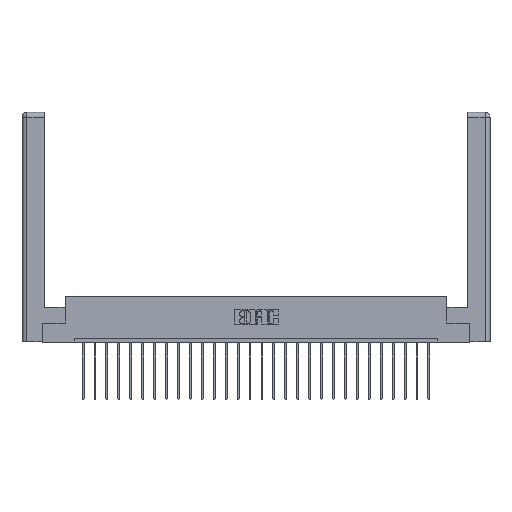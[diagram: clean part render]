
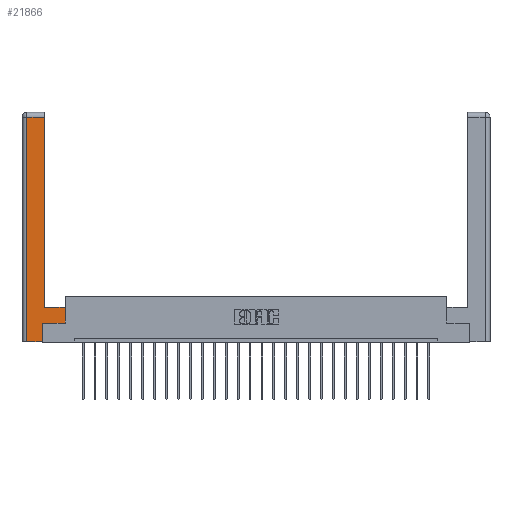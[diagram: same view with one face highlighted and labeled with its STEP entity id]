
A CAD part, top view. The second image highlights one B-rep face of the part: STEP entity #21866.
In plain terms, the highlighted planar face has unit normal (0, 0, 1).
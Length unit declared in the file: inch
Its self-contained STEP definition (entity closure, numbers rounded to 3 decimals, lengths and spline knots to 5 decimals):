
#73 = EDGE_CURVE ( 'NONE', #23900, #25314, #4534, .T. ) ;
#271 = CARTESIAN_POINT ( 'NONE',  ( 0.295, 0.45, 0. ) ) ;
#845 = VECTOR ( 'NONE', #26186, 39.37008 ) ;
#1394 = EDGE_LOOP ( 'NONE', ( #19940, #19901, #8813, #25549, #12330, #16072, #11205, #23331 ) ) ;
#1523 = CARTESIAN_POINT ( 'NONE',  ( 0.565, 0.245, 0. ) ) ;
#1607 = AXIS2_PLACEMENT_3D ( 'NONE', #14791, #22814, #22998 ) ;
#3535 = CARTESIAN_POINT ( 'NONE',  ( 0.265, 0.245, 0. ) ) ;
#4013 = DIRECTION ( 'NONE',  ( -1., 0., 0. ) ) ;
#4534 = LINE ( 'NONE', #16246, #7686 ) ;
#4555 = VECTOR ( 'NONE', #17976, 39.37008 ) ;
#5051 = EDGE_CURVE ( 'NONE', #6829, #8769, #17797, .T. ) ;
#5278 = EDGE_CURVE ( 'NONE', #17995, #23900, #6553, .T. ) ;
#5925 = DIRECTION ( 'NONE',  ( 0., 1., 0. ) ) ;
#6553 = LINE ( 'NONE', #7873, #16489 ) ;
#6637 = VECTOR ( 'NONE', #18318, 39.37008 ) ;
#6829 = VERTEX_POINT ( 'NONE', #17861 ) ;
#7098 = CARTESIAN_POINT ( 'NONE',  ( 0.265, 0., 0. ) ) ;
#7109 = EDGE_CURVE ( 'NONE', #25314, #8483, #14749, .T. ) ;
#7280 = LINE ( 'NONE', #13792, #18877 ) ;
#7686 = VECTOR ( 'NONE', #4013, 39.37008 ) ;
#7867 = CARTESIAN_POINT ( 'NONE',  ( 0.0615, 2.94, 0. ) ) ;
#7873 = CARTESIAN_POINT ( 'NONE',  ( 0.565, 0.45, 0. ) ) ;
#8245 = CARTESIAN_POINT ( 'NONE',  ( 0.0615, 2.94, 0. ) ) ;
#8483 = VERTEX_POINT ( 'NONE', #11655 ) ;
#8769 = VERTEX_POINT ( 'NONE', #7098 ) ;
#8813 = ORIENTED_EDGE ( 'NONE', *, *, #12020, .T. ) ;
#9051 = EDGE_CURVE ( 'NONE', #8483, #21512, #10827, .T. ) ;
#9199 = DIRECTION ( 'NONE',  ( 0., 1., 0. ) ) ;
#10827 = LINE ( 'NONE', #8245, #6637 ) ;
#10844 = CARTESIAN_POINT ( 'NONE',  ( 0.295, 3., 0. ) ) ;
#11021 = LINE ( 'NONE', #13628, #20618 ) ;
#11205 = ORIENTED_EDGE ( 'NONE', *, *, #5278, .T. ) ;
#11655 = CARTESIAN_POINT ( 'NONE',  ( 0.295, 2.94, 0. ) ) ;
#12020 = EDGE_CURVE ( 'NONE', #21512, #6829, #11021, .T. ) ;
#12039 = CARTESIAN_POINT ( 'NONE',  ( 0.565, 0.45, 0. ) ) ;
#12330 = ORIENTED_EDGE ( 'NONE', *, *, #20867, .T. ) ;
#13628 = CARTESIAN_POINT ( 'NONE',  ( 0.0615, 0., 0. ) ) ;
#13792 = CARTESIAN_POINT ( 'NONE',  ( 0.265, 0.245, 0. ) ) ;
#13801 = DIRECTION ( 'NONE',  ( 0., -1., 0. ) ) ;
#13814 = LINE ( 'NONE', #1523, #4555 ) ;
#14749 = LINE ( 'NONE', #10844, #19306 ) ;
#14791 = CARTESIAN_POINT ( 'NONE',  ( 0., 0., 0. ) ) ;
#15151 = VERTEX_POINT ( 'NONE', #3535 ) ;
#16072 = ORIENTED_EDGE ( 'NONE', *, *, #20217, .T. ) ;
#16246 = CARTESIAN_POINT ( 'NONE',  ( 0.295, 0.45, 0. ) ) ;
#16286 = CARTESIAN_POINT ( 'NONE',  ( 0.265, 0., 0. ) ) ;
#16489 = VECTOR ( 'NONE', #24503, 39.37008 ) ;
#16873 = FACE_OUTER_BOUND ( 'NONE', #1394, .T. ) ;
#17797 = LINE ( 'NONE', #16286, #845 ) ;
#17861 = CARTESIAN_POINT ( 'NONE',  ( 0.0615, 0., 0. ) ) ;
#17976 = DIRECTION ( 'NONE',  ( 1., 0., 0. ) ) ;
#17995 = VERTEX_POINT ( 'NONE', #21068 ) ;
#18318 = DIRECTION ( 'NONE',  ( -1., 0., 0. ) ) ;
#18877 = VECTOR ( 'NONE', #5925, 39.37008 ) ;
#19306 = VECTOR ( 'NONE', #9199, 39.37008 ) ;
#19901 = ORIENTED_EDGE ( 'NONE', *, *, #9051, .T. ) ;
#19940 = ORIENTED_EDGE ( 'NONE', *, *, #7109, .T. ) ;
#20217 = EDGE_CURVE ( 'NONE', #15151, #17995, #13814, .T. ) ;
#20618 = VECTOR ( 'NONE', #13801, 39.37008 ) ;
#20867 = EDGE_CURVE ( 'NONE', #8769, #15151, #7280, .T. ) ;
#21068 = CARTESIAN_POINT ( 'NONE',  ( 0.565, 0.245, 0. ) ) ;
#21512 = VERTEX_POINT ( 'NONE', #7867 ) ;
#21866 = ADVANCED_FACE ( 'NONE', ( #16873 ), #24896, .F. ) ;
#22814 = DIRECTION ( 'NONE',  ( 0., 0., -1. ) ) ;
#22998 = DIRECTION ( 'NONE',  ( -1., 0., 0. ) ) ;
#23331 = ORIENTED_EDGE ( 'NONE', *, *, #73, .T. ) ;
#23900 = VERTEX_POINT ( 'NONE', #12039 ) ;
#24503 = DIRECTION ( 'NONE',  ( 0., 1., 0. ) ) ;
#24896 = PLANE ( 'NONE',  #1607 ) ;
#25314 = VERTEX_POINT ( 'NONE', #271 ) ;
#25549 = ORIENTED_EDGE ( 'NONE', *, *, #5051, .T. ) ;
#26186 = DIRECTION ( 'NONE',  ( 1., 0., 0. ) ) ;
